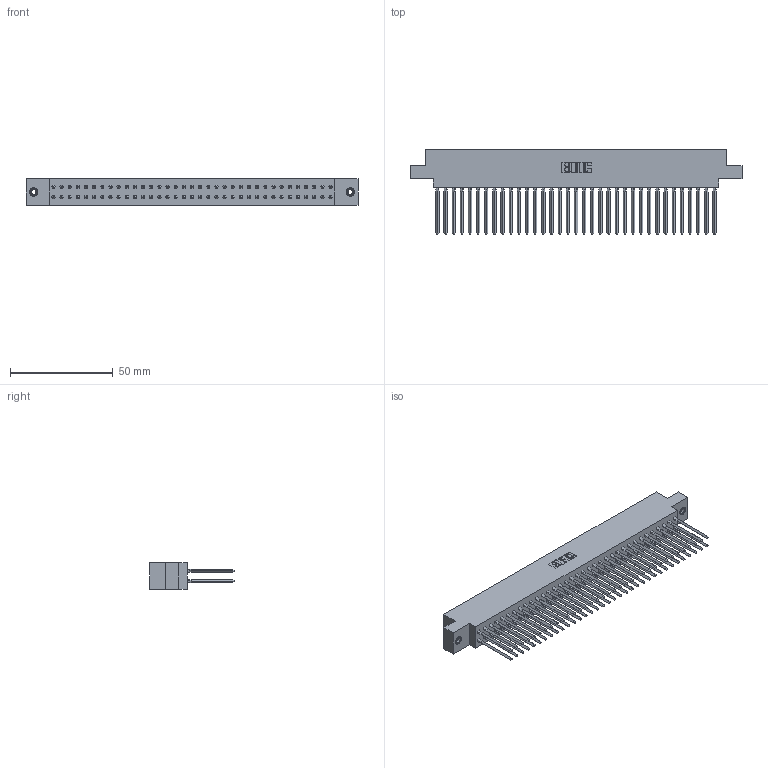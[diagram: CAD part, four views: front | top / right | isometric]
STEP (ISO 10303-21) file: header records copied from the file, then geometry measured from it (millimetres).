
FILE_DESCRIPTION (( 'STEP AP203' ), '1' );
FILE_NAME ('317-070-543-878.STEP', '2020-02-28T07:19:51', ( '' ), ( '' ), 'SwSTEP 2.0', 'SolidWorks 2016', '' );
FILE_SCHEMA (( 'CONFIG_CONTROL_DESIGN' ));
Length unit declared in the file: inch
Products named in the file (4): 317 Part_.156 Dia - TI; 345-250-001_345-250-003-102; 317-290-001_543; 317-070-543-878
Assembly tree (73 placements, depth 2):
  317-070-543-878
    317 Part_.156 Dia - TI
    317-290-001_543  x70
    345-250-001_345-250-003-102  x2
Bounding box: 161.39 x 41.15 x 12.7 mm (x, y, z)
Volume: 27191.7 mm3; surface area: 40998.2 mm2
Topology: 73 solids, 73 shells, 6392 faces, 17701 edges, 11396 vertices
Faces by surface type: plane 5200, cylinder 896, bspline 280, cone 12, torus 4
Entity records: 52755 total; most frequent: CARTESIAN_POINT 9590, ORIENTED_EDGE 9082, DIRECTION 7617, EDGE_CURVE 4541, VECTOR 4265, LINE 4265, VERTEX_POINT 3017, AXIS2_PLACEMENT_3D 1676
